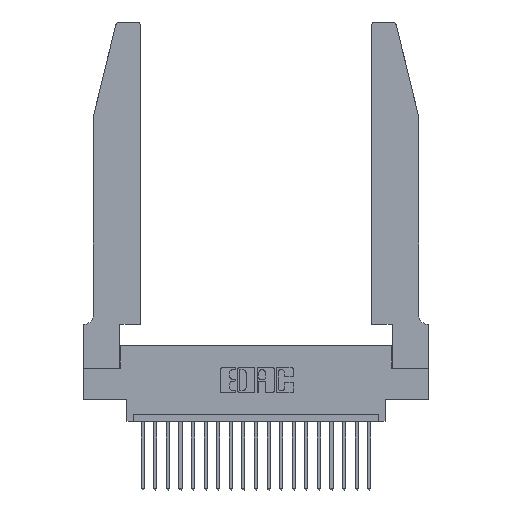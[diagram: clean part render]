
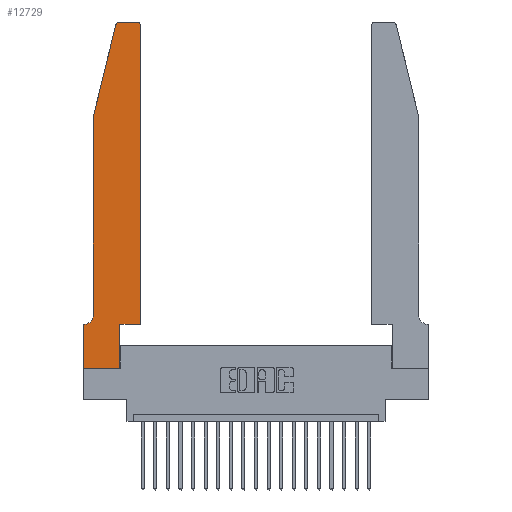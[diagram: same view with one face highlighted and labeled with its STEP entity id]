
A CAD part, top view. The second image highlights one B-rep face of the part: STEP entity #12729.
In plain terms, the highlighted planar face has unit normal (0, 0, 1).
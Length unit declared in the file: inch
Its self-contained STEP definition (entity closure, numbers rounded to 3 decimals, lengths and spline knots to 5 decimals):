
#450 = VERTEX_POINT ( 'NONE', #13079 ) ;
#646 = CARTESIAN_POINT ( 'NONE',  ( 0.0755, 2., 0.37 ) ) ;
#826 = CARTESIAN_POINT ( 'NONE',  ( 0.25487, 2.72718, 0.37 ) ) ;
#1055 = EDGE_CURVE ( 'NONE', #15544, #13003, #6104, .T. ) ;
#1241 = VECTOR ( 'NONE', #18507, 39.37008 ) ;
#1652 = CARTESIAN_POINT ( 'NONE',  ( 0.4205, 2.75, 0.37 ) ) ;
#1691 = DIRECTION ( 'NONE',  ( 1., 0., 0. ) ) ;
#1753 = DIRECTION ( 'NONE',  ( 1., 0., 0. ) ) ;
#1924 = EDGE_CURVE ( 'NONE', #17363, #5858, #17392, .T. ) ;
#2032 = DIRECTION ( 'NONE',  ( 0., -1., 0. ) ) ;
#2288 = EDGE_LOOP ( 'NONE', ( #7956, #10081, #2733, #14600, #10995, #2972, #14857, #22252, #10616, #11579, #13902, #10952 ) ) ;
#2342 = LINE ( 'NONE', #9989, #19054 ) ;
#2381 = CARTESIAN_POINT ( 'NONE',  ( 0.0055, 0.42, 0.37 ) ) ;
#2385 = CARTESIAN_POINT ( 'NONE',  ( 0.284, 2.72, 0.37 ) ) ;
#2396 = LINE ( 'NONE', #12549, #21247 ) ;
#2537 = AXIS2_PLACEMENT_3D ( 'NONE', #2385, #12754, #17745 ) ;
#2670 = VERTEX_POINT ( 'NONE', #18524 ) ;
#2733 = ORIENTED_EDGE ( 'NONE', *, *, #10030, .T. ) ;
#2972 = ORIENTED_EDGE ( 'NONE', *, *, #1924, .T. ) ;
#3912 = CARTESIAN_POINT ( 'NONE',  ( 0.4505, 2.72, 0.37 ) ) ;
#3921 = LINE ( 'NONE', #12348, #7932 ) ;
#3989 = DIRECTION ( 'NONE',  ( 0., 1., 0. ) ) ;
#4055 = DIRECTION ( 'NONE',  ( 0., -1., 0. ) ) ;
#5046 = VERTEX_POINT ( 'NONE', #826 ) ;
#5091 = CARTESIAN_POINT ( 'NONE',  ( 0.4205, 2.72, 0.37 ) ) ;
#5814 = DIRECTION ( 'NONE',  ( -1., 0., 0. ) ) ;
#5858 = VERTEX_POINT ( 'NONE', #22167 ) ;
#6104 = CIRCLE ( 'NONE', #20055, 0.03 ) ;
#6382 = VERTEX_POINT ( 'NONE', #8381 ) ;
#6392 = VERTEX_POINT ( 'NONE', #12585 ) ;
#6444 = CARTESIAN_POINT ( 'NONE',  ( 0.4505, 0.35, 0.37 ) ) ;
#6465 = PLANE ( 'NONE',  #17420 ) ;
#6615 = DIRECTION ( 'NONE',  ( 0., 0., 1. ) ) ;
#6955 = DIRECTION ( 'NONE',  ( 1., 0., 0. ) ) ;
#7737 = CARTESIAN_POINT ( 'NONE',  ( 0.4505, 0.35, 0.37 ) ) ;
#7770 = VERTEX_POINT ( 'NONE', #19272 ) ;
#7774 = LINE ( 'NONE', #17787, #10988 ) ;
#7932 = VECTOR ( 'NONE', #2032, 39.37008 ) ;
#7956 = ORIENTED_EDGE ( 'NONE', *, *, #9075, .T. ) ;
#8116 = VECTOR ( 'NONE', #6955, 39.37008 ) ;
#8381 = CARTESIAN_POINT ( 'NONE',  ( 0.2865, 0., 0.37 ) ) ;
#8412 = CARTESIAN_POINT ( 'NONE',  ( 0., 0., 0.37 ) ) ;
#8883 = EDGE_CURVE ( 'NONE', #2670, #5046, #10801, .T. ) ;
#8899 = EDGE_CURVE ( 'NONE', #6392, #7770, #19456, .T. ) ;
#8932 = DIRECTION ( 'NONE',  ( -1., 0., 0. ) ) ;
#9075 = EDGE_CURVE ( 'NONE', #13003, #2670, #20522, .T. ) ;
#9180 = VECTOR ( 'NONE', #4055, 39.37008 ) ;
#9617 = CIRCLE ( 'NONE', #14815, 0.07 ) ;
#9989 = CARTESIAN_POINT ( 'NONE',  ( 0., 0., 0.37 ) ) ;
#10030 = EDGE_CURVE ( 'NONE', #5046, #6392, #7774, .T. ) ;
#10081 = ORIENTED_EDGE ( 'NONE', *, *, #8883, .T. ) ;
#10338 = CARTESIAN_POINT ( 'NONE',  ( 0.2605, 2.75, 0.37 ) ) ;
#10553 = VERTEX_POINT ( 'NONE', #14461 ) ;
#10616 = ORIENTED_EDGE ( 'NONE', *, *, #15526, .T. ) ;
#10801 = CIRCLE ( 'NONE', #2537, 0.03 ) ;
#10827 = LINE ( 'NONE', #7737, #8116 ) ;
#10952 = ORIENTED_EDGE ( 'NONE', *, *, #1055, .T. ) ;
#10988 = VECTOR ( 'NONE', #19554, 39.37008 ) ;
#10995 = ORIENTED_EDGE ( 'NONE', *, *, #11239, .T. ) ;
#11195 = EDGE_CURVE ( 'NONE', #12545, #6382, #2342, .T. ) ;
#11239 = EDGE_CURVE ( 'NONE', #7770, #17363, #9617, .T. ) ;
#11579 = ORIENTED_EDGE ( 'NONE', *, *, #13329, .T. ) ;
#11728 = VECTOR ( 'NONE', #8932, 39.37008 ) ;
#12264 = EDGE_CURVE ( 'NONE', #5858, #12545, #3921, .T. ) ;
#12348 = CARTESIAN_POINT ( 'NONE',  ( 0., 0., 0.37 ) ) ;
#12545 = VERTEX_POINT ( 'NONE', #8412 ) ;
#12549 = CARTESIAN_POINT ( 'NONE',  ( 0.2865, 0.35, 0.37 ) ) ;
#12585 = CARTESIAN_POINT ( 'NONE',  ( 0.0755, 2., 0.37 ) ) ;
#12729 = ADVANCED_FACE ( 'NONE', ( #22142 ), #6465, .T. ) ;
#12754 = DIRECTION ( 'NONE',  ( 0., 0., 1. ) ) ;
#13003 = VERTEX_POINT ( 'NONE', #1652 ) ;
#13079 = CARTESIAN_POINT ( 'NONE',  ( 0.4505, 0.35, 0.37 ) ) ;
#13329 = EDGE_CURVE ( 'NONE', #10553, #450, #10827, .T. ) ;
#13902 = ORIENTED_EDGE ( 'NONE', *, *, #16689, .T. ) ;
#14461 = CARTESIAN_POINT ( 'NONE',  ( 0.2865, 0.35, 0.37 ) ) ;
#14600 = ORIENTED_EDGE ( 'NONE', *, *, #8899, .T. ) ;
#14815 = AXIS2_PLACEMENT_3D ( 'NONE', #2381, #19340, #5814 ) ;
#14857 = ORIENTED_EDGE ( 'NONE', *, *, #12264, .T. ) ;
#15526 = EDGE_CURVE ( 'NONE', #6382, #10553, #2396, .T. ) ;
#15544 = VERTEX_POINT ( 'NONE', #3912 ) ;
#15936 = VECTOR ( 'NONE', #19726, 39.37008 ) ;
#16689 = EDGE_CURVE ( 'NONE', #450, #15544, #18756, .T. ) ;
#16872 = CARTESIAN_POINT ( 'NONE',  ( 0., 0.35, 0.37 ) ) ;
#17008 = DIRECTION ( 'NONE',  ( 1., 0., 0. ) ) ;
#17319 = CARTESIAN_POINT ( 'NONE',  ( 0.0055, 0.35, 0.37 ) ) ;
#17363 = VERTEX_POINT ( 'NONE', #17319 ) ;
#17392 = LINE ( 'NONE', #17850, #11728 ) ;
#17420 = AXIS2_PLACEMENT_3D ( 'NONE', #16872, #6615, #1753 ) ;
#17745 = DIRECTION ( 'NONE',  ( 1., 0., 0. ) ) ;
#17787 = CARTESIAN_POINT ( 'NONE',  ( 0.0755, 2., 0.37 ) ) ;
#17850 = CARTESIAN_POINT ( 'NONE',  ( 0.0755, 0.35, 0.37 ) ) ;
#18507 = DIRECTION ( 'NONE',  ( 0., 1., 0. ) ) ;
#18524 = CARTESIAN_POINT ( 'NONE',  ( 0.284, 2.75, 0.37 ) ) ;
#18756 = LINE ( 'NONE', #6444, #1241 ) ;
#19054 = VECTOR ( 'NONE', #17008, 39.37008 ) ;
#19272 = CARTESIAN_POINT ( 'NONE',  ( 0.0755, 0.42, 0.37 ) ) ;
#19340 = DIRECTION ( 'NONE',  ( 0., 0., -1. ) ) ;
#19456 = LINE ( 'NONE', #646, #9180 ) ;
#19554 = DIRECTION ( 'NONE',  ( -0.239, -0.971, 0. ) ) ;
#19726 = DIRECTION ( 'NONE',  ( -1., 0., 0. ) ) ;
#20055 = AXIS2_PLACEMENT_3D ( 'NONE', #5091, #20751, #1691 ) ;
#20522 = LINE ( 'NONE', #10338, #15936 ) ;
#20751 = DIRECTION ( 'NONE',  ( 0., 0., 1. ) ) ;
#21247 = VECTOR ( 'NONE', #3989, 39.37008 ) ;
#22142 = FACE_OUTER_BOUND ( 'NONE', #2288, .T. ) ;
#22167 = CARTESIAN_POINT ( 'NONE',  ( 0., 0.35, 0.37 ) ) ;
#22252 = ORIENTED_EDGE ( 'NONE', *, *, #11195, .T. ) ;
